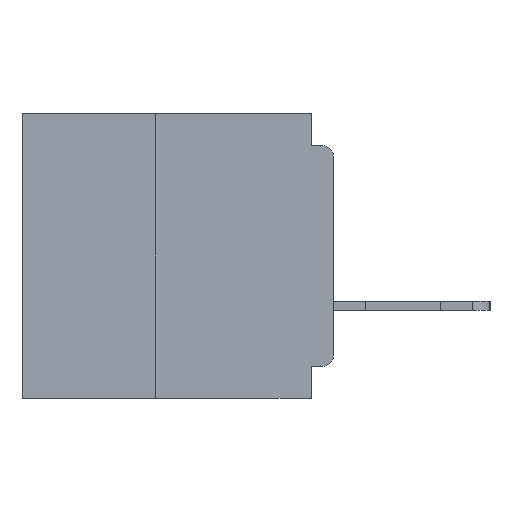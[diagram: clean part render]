
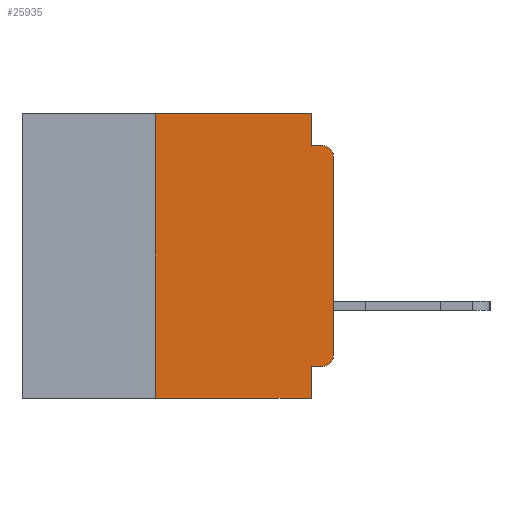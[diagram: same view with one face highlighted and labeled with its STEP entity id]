
A CAD part, left-side view. The second image highlights one B-rep face of the part: STEP entity #25935.
In plain terms, the highlighted planar face has unit normal (-1, 0, 0).
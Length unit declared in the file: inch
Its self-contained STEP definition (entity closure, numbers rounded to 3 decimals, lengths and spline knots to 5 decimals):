
#473 = LINE ( 'NONE', #31482, #1444 ) ;
#1444 = VECTOR ( 'NONE', #10454, 39.37008 ) ;
#1537 = DIRECTION ( 'NONE',  ( 0., 0., -1. ) ) ;
#2507 = DIRECTION ( 'NONE',  ( 0., 0., -1. ) ) ;
#2830 = CARTESIAN_POINT ( 'NONE',  ( 0., 0.015, -0.34 ) ) ;
#2979 = EDGE_CURVE ( 'NONE', #20500, #13719, #18623, .T. ) ;
#3161 = DIRECTION ( 'NONE',  ( 0., -1., 0. ) ) ;
#3216 = DIRECTION ( 'NONE',  ( 0., 0., 1. ) ) ;
#3968 = EDGE_CURVE ( 'NONE', #35204, #35390, #14806, .T. ) ;
#4067 = VERTEX_POINT ( 'NONE', #10723 ) ;
#4232 = ORIENTED_EDGE ( 'NONE', *, *, #2979, .T. ) ;
#5375 = ORIENTED_EDGE ( 'NONE', *, *, #6020, .F. ) ;
#5443 = CARTESIAN_POINT ( 'NONE',  ( 0., 0.015, -0.355 ) ) ;
#5907 = DIRECTION ( 'NONE',  ( 0., 0., -1. ) ) ;
#6020 = EDGE_CURVE ( 'NONE', #35204, #31001, #9022, .T. ) ;
#6043 = ORIENTED_EDGE ( 'NONE', *, *, #34048, .T. ) ;
#6254 = VECTOR ( 'NONE', #3216, 39.37008 ) ;
#6649 = DIRECTION ( 'NONE',  ( 1., 0., 0. ) ) ;
#6857 = LINE ( 'NONE', #17618, #37936 ) ;
#7099 = EDGE_CURVE ( 'NONE', #37522, #28560, #28507, .T. ) ;
#8097 = EDGE_CURVE ( 'NONE', #4067, #38582, #473, .T. ) ;
#8392 = EDGE_CURVE ( 'NONE', #20020, #20500, #14330, .T. ) ;
#9022 = LINE ( 'NONE', #38424, #32081 ) ;
#9456 = PLANE ( 'NONE',  #22916 ) ;
#9566 = EDGE_LOOP ( 'NONE', ( #38618, #4232, #35690, #13525, #24043, #5375, #22827, #35179, #24612, #6043 ) ) ;
#9621 = VECTOR ( 'NONE', #21075, 39.37008 ) ;
#10194 = CARTESIAN_POINT ( 'NONE',  ( 0., 0.437, -0.4 ) ) ;
#10454 = DIRECTION ( 'NONE',  ( 0., 0., -1. ) ) ;
#10723 = CARTESIAN_POINT ( 'NONE',  ( 0., 0.031, 0. ) ) ;
#11514 = DIRECTION ( 'NONE',  ( 0., 0., 1. ) ) ;
#12103 = CARTESIAN_POINT ( 'NONE',  ( 0., 0.25, -0.4 ) ) ;
#12632 = CARTESIAN_POINT ( 'NONE',  ( 0., 0.437, 0. ) ) ;
#12934 = VECTOR ( 'NONE', #22115, 39.37008 ) ;
#13504 = VECTOR ( 'NONE', #23217, 39.37008 ) ;
#13525 = ORIENTED_EDGE ( 'NONE', *, *, #8097, .F. ) ;
#13719 = VERTEX_POINT ( 'NONE', #34160 ) ;
#14331 = CARTESIAN_POINT ( 'NONE',  ( 0., 0., -0.355 ) ) ;
#14330 = LINE ( 'NONE', #27234, #6254 ) ;
#14806 = LINE ( 'NONE', #10194, #12934 ) ;
#16046 = FACE_OUTER_BOUND ( 'NONE', #9566, .T. ) ;
#17618 = CARTESIAN_POINT ( 'NONE',  ( 0., 0.031, -0.4 ) ) ;
#17745 = CARTESIAN_POINT ( 'NONE',  ( 0., 0.031, -0.045 ) ) ;
#18066 = CARTESIAN_POINT ( 'NONE',  ( 0., 0.437, 0. ) ) ;
#18530 = LINE ( 'NONE', #18066, #9621 ) ;
#18623 = CIRCLE ( 'NONE', #24330, 0.015 ) ;
#19705 = DIRECTION ( 'NONE',  ( -1., 0., 0. ) ) ;
#20020 = VERTEX_POINT ( 'NONE', #30593 ) ;
#20500 = VERTEX_POINT ( 'NONE', #27105 ) ;
#21075 = DIRECTION ( 'NONE',  ( 0., -1., 0. ) ) ;
#21246 = CARTESIAN_POINT ( 'NONE',  ( 0., 0., -0.045 ) ) ;
#22115 = DIRECTION ( 'NONE',  ( 0., -1., 0. ) ) ;
#22827 = ORIENTED_EDGE ( 'NONE', *, *, #3968, .T. ) ;
#22916 = AXIS2_PLACEMENT_3D ( 'NONE', #12632, #6649, #27706 ) ;
#23217 = DIRECTION ( 'NONE',  ( 0., 1., 0. ) ) ;
#23938 = DIRECTION ( 'NONE',  ( -1., 0., 0. ) ) ;
#24043 = ORIENTED_EDGE ( 'NONE', *, *, #32610, .F. ) ;
#24330 = AXIS2_PLACEMENT_3D ( 'NONE', #37728, #19705, #1537 ) ;
#24612 = ORIENTED_EDGE ( 'NONE', *, *, #7099, .F. ) ;
#25918 = CIRCLE ( 'NONE', #37520, 0.015 ) ;
#25935 = ADVANCED_FACE ( 'NONE', ( #16046 ), #9456, .F. ) ;
#27105 = CARTESIAN_POINT ( 'NONE',  ( 0., 0., -0.06 ) ) ;
#27234 = CARTESIAN_POINT ( 'NONE',  ( 0., 0., 0. ) ) ;
#27257 = EDGE_CURVE ( 'NONE', #38582, #13719, #37081, .T. ) ;
#27706 = DIRECTION ( 'NONE',  ( 0., 0., -1. ) ) ;
#28507 = LINE ( 'NONE', #14331, #13504 ) ;
#28560 = VERTEX_POINT ( 'NONE', #31042 ) ;
#30034 = VECTOR ( 'NONE', #3161, 39.37008 ) ;
#30593 = CARTESIAN_POINT ( 'NONE',  ( 0., 0., -0.34 ) ) ;
#30998 = CARTESIAN_POINT ( 'NONE',  ( 0., 0.031, -0.4 ) ) ;
#31001 = VERTEX_POINT ( 'NONE', #36978 ) ;
#31042 = CARTESIAN_POINT ( 'NONE',  ( 0., 0.031, -0.355 ) ) ;
#31482 = CARTESIAN_POINT ( 'NONE',  ( 0., 0.031, 0. ) ) ;
#32081 = VECTOR ( 'NONE', #11514, 39.37008 ) ;
#32610 = EDGE_CURVE ( 'NONE', #31001, #4067, #18530, .T. ) ;
#34048 = EDGE_CURVE ( 'NONE', #37522, #20020, #25918, .T. ) ;
#34160 = CARTESIAN_POINT ( 'NONE',  ( 0., 0.015, -0.045 ) ) ;
#35179 = ORIENTED_EDGE ( 'NONE', *, *, #37048, .F. ) ;
#35204 = VERTEX_POINT ( 'NONE', #12103 ) ;
#35390 = VERTEX_POINT ( 'NONE', #30998 ) ;
#35690 = ORIENTED_EDGE ( 'NONE', *, *, #27257, .F. ) ;
#36978 = CARTESIAN_POINT ( 'NONE',  ( 0., 0.25, 0. ) ) ;
#37048 = EDGE_CURVE ( 'NONE', #28560, #35390, #6857, .T. ) ;
#37081 = LINE ( 'NONE', #21246, #30034 ) ;
#37520 = AXIS2_PLACEMENT_3D ( 'NONE', #2830, #23938, #5907 ) ;
#37522 = VERTEX_POINT ( 'NONE', #5443 ) ;
#37728 = CARTESIAN_POINT ( 'NONE',  ( 0., 0.015, -0.06 ) ) ;
#37936 = VECTOR ( 'NONE', #2507, 39.37008 ) ;
#38424 = CARTESIAN_POINT ( 'NONE',  ( 0., 0.25, -0.4 ) ) ;
#38582 = VERTEX_POINT ( 'NONE', #17745 ) ;
#38618 = ORIENTED_EDGE ( 'NONE', *, *, #8392, .T. ) ;
